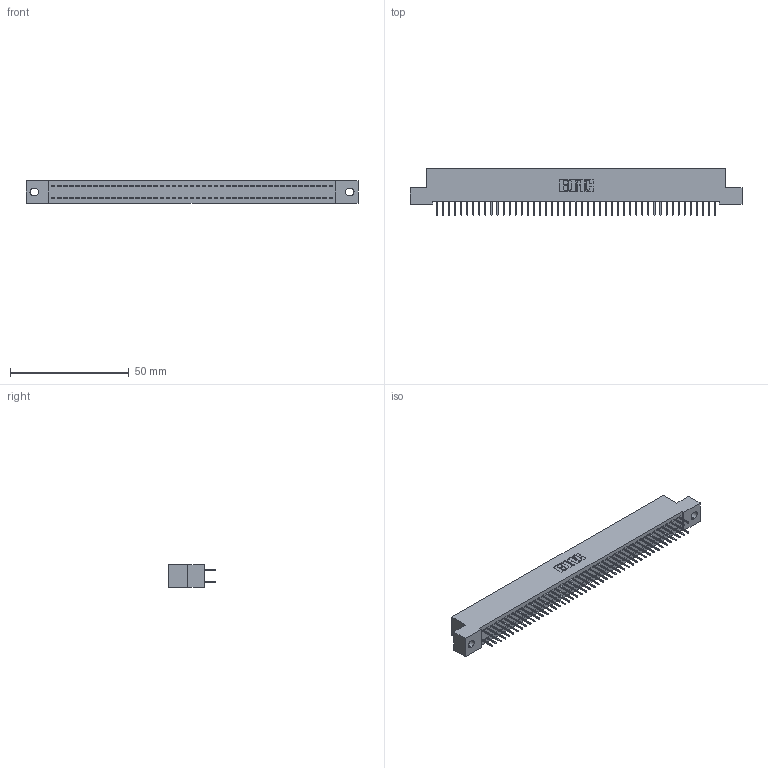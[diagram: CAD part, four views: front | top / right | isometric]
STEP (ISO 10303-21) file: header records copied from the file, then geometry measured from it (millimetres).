
FILE_DESCRIPTION (( 'STEP AP203' ), '1' );
FILE_NAME ('392-094-524-202.STEP', '2019-10-09T19:17:59', ( '' ), ( '' ), 'SwSTEP 2.0', 'SolidWorks 2016', '' );
FILE_SCHEMA (( 'CONFIG_CONTROL_DESIGN' ));
Length unit declared in the file: inch
Products named in the file (3): 342 Part_.128 Slot; 345-292-001_345-293-124; 392-094-524-202
Assembly tree (95 placements, depth 2):
  392-094-524-202
    342 Part_.128 Slot
    345-292-001_345-293-124  x94
Bounding box: 139.7 x 19.69 x 9.4 mm (x, y, z)
Volume: 12381.3 mm3; surface area: 19666.3 mm2
Topology: 95 solids, 95 shells, 5378 faces, 15257 edges, 9794 vertices
Faces by surface type: plane 4018, cylinder 1360
Entity records: 29667 total; most frequent: CARTESIAN_POINT 4910, ORIENTED_EDGE 4846, DIRECTION 4187, EDGE_CURVE 2423, VECTOR 2299, LINE 2299, VERTEX_POINT 1610, AXIS2_PLACEMENT_3D 944
